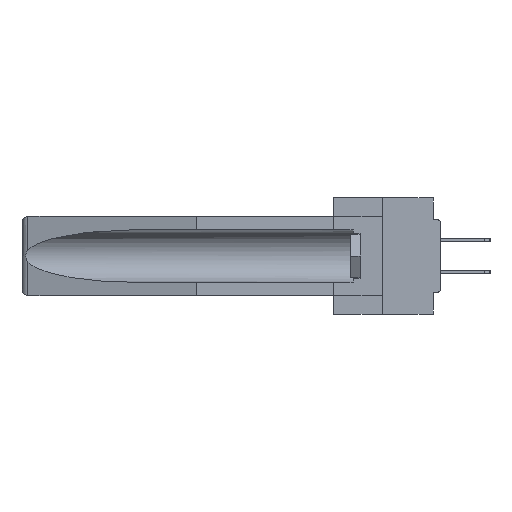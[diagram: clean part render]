
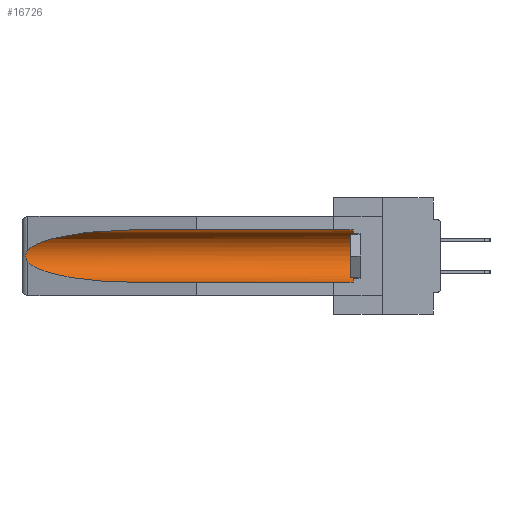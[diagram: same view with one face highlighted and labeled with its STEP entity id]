
A CAD part, left-side view. The second image highlights one B-rep face of the part: STEP entity #16726.
In plain terms, the highlighted cylindrical face has radius 2.857 mm (diameter 5.715 mm), a partial arc.
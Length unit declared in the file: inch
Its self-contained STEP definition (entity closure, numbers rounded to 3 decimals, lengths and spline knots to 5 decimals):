
#1860 = CARTESIAN_POINT ( 'NONE',  ( 0.2675, 1.53308, -0.16763 ) ) ;
#2304 = DIRECTION ( 'NONE',  ( 0., 1., 0. ) ) ;
#3188 = CARTESIAN_POINT ( 'NONE',  ( 0.25451, 1.48313, -0.09465 ) ) ;
#3666 = CARTESIAN_POINT ( 'NONE',  ( 0.155, 1.07973, -0.059 ) ) ;
#4475 = CARTESIAN_POINT ( 'NONE',  ( 0.26537, 1.52718, -0.19328 ) ) ;
#4611 = CARTESIAN_POINT ( 'NONE',  ( 0.26537, 1.52718, -0.14972 ) ) ;
#4769 = VERTEX_POINT ( 'NONE', #35009 ) ;
#4998 = AXIS2_PLACEMENT_3D ( 'NONE', #13197, #9573, #36963 ) ;
#6229 =( BOUNDED_CURVE ( )  B_SPLINE_CURVE ( 3, ( #36138, #35714, #3188, #15961 ),
 .UNSPECIFIED., .F., .F. ) 
 B_SPLINE_CURVE_WITH_KNOTS ( ( 4, 4 ),
 ( 4.71239, 6.08839 ),
 .UNSPECIFIED. ) 
 CURVE ( )  GEOMETRIC_REPRESENTATION_ITEM ( )  RATIONAL_B_SPLINE_CURVE ( ( 1., 0.848, 0.848, 1. ) ) 
 REPRESENTATION_ITEM ( '' )  );
#6712 = DIRECTION ( 'NONE',  ( 0., -1., 0. ) ) ;
#7484 = LINE ( 'NONE', #21594, #15284 ) ;
#8739 = VERTEX_POINT ( 'NONE', #35648 ) ;
#9002 = CARTESIAN_POINT ( 'NONE',  ( 0.21114, 1.30732, -0.284 ) ) ;
#9573 = DIRECTION ( 'NONE',  ( 0., 1., 0. ) ) ;
#9753 = ORIENTED_EDGE ( 'NONE', *, *, #20040, .T. ) ;
#10214 =( BOUNDED_CURVE ( )  B_SPLINE_CURVE ( 3, ( #25278, #19764, #9002, #38895 ),
 .UNSPECIFIED., .F., .F. ) 
 B_SPLINE_CURVE_WITH_KNOTS ( ( 4, 4 ),
 ( 0.1948, 1.5708 ),
 .UNSPECIFIED. ) 
 CURVE ( )  GEOMETRIC_REPRESENTATION_ITEM ( )  RATIONAL_B_SPLINE_CURVE ( ( 1., 0.848, 0.848, 1. ) ) 
 REPRESENTATION_ITEM ( '' )  );
#11291 = CARTESIAN_POINT ( 'NONE',  ( 0.2675, 1.53308, -0.17534 ) ) ;
#13197 = CARTESIAN_POINT ( 'NONE',  ( 0.155, -0.30754, -0.1715 ) ) ;
#14502 = ORIENTED_EDGE ( 'NONE', *, *, #35498, .T. ) ;
#15072 = CARTESIAN_POINT ( 'NONE',  ( 0.155, -0.30754, -0.059 ) ) ;
#15284 = VECTOR ( 'NONE', #37813, 39.37008 ) ;
#15778 = EDGE_LOOP ( 'NONE', ( #18957, #9753, #29349, #20083, #36887, #14502 ) ) ;
#15961 = CARTESIAN_POINT ( 'NONE',  ( 0.26537, 1.52718, -0.14972 ) ) ;
#16284 = EDGE_CURVE ( 'NONE', #30520, #24343, #24476, .T. ) ;
#16726 = ADVANCED_FACE ( 'NONE', ( #35346 ), #37397, .F. ) ;
#18957 = ORIENTED_EDGE ( 'NONE', *, *, #32190, .T. ) ;
#18969 = CARTESIAN_POINT ( 'NONE',  ( 0.155, 0.126, -0.284 ) ) ;
#19764 = CARTESIAN_POINT ( 'NONE',  ( 0.25451, 1.48313, -0.24835 ) ) ;
#20040 = EDGE_CURVE ( 'NONE', #4769, #8739, #41049, .T. ) ;
#20083 = ORIENTED_EDGE ( 'NONE', *, *, #35715, .F. ) ;
#21594 = CARTESIAN_POINT ( 'NONE',  ( 0.155, -0.30754, -0.284 ) ) ;
#24343 = VERTEX_POINT ( 'NONE', #40068 ) ;
#24476 = CIRCLE ( 'NONE', #41705, 0.1125 ) ;
#24818 = CARTESIAN_POINT ( 'NONE',  ( 0.26597, 1.5296, -0.19026 ) ) ;
#25278 = CARTESIAN_POINT ( 'NONE',  ( 0.26537, 1.52718, -0.19328 ) ) ;
#26588 = CARTESIAN_POINT ( 'NONE',  ( 0.155, 0.126, -0.1715 ) ) ;
#29349 = ORIENTED_EDGE ( 'NONE', *, *, #31550, .T. ) ;
#29413 = VERTEX_POINT ( 'NONE', #42694 ) ;
#29922 = DIRECTION ( 'NONE',  ( 0., 0., 1. ) ) ;
#30520 = VERTEX_POINT ( 'NONE', #18969 ) ;
#31341 = CARTESIAN_POINT ( 'NONE',  ( 0.2673, 1.53269, -0.17917 ) ) ;
#31491 = CARTESIAN_POINT ( 'NONE',  ( 0.26654, 1.53092, -0.15636 ) ) ;
#31550 = EDGE_CURVE ( 'NONE', #8739, #29413, #10214, .T. ) ;
#32190 = EDGE_CURVE ( 'NONE', #40282, #4769, #6229, .T. ) ;
#32474 = LINE ( 'NONE', #15072, #40699 ) ;
#34662 = CARTESIAN_POINT ( 'NONE',  ( 0.26655, 1.53094, -0.18657 ) ) ;
#35009 = CARTESIAN_POINT ( 'NONE',  ( 0.26537, 1.52718, -0.14972 ) ) ;
#35346 = FACE_OUTER_BOUND ( 'NONE', #15778, .T. ) ;
#35498 = EDGE_CURVE ( 'NONE', #24343, #40282, #32474, .T. ) ;
#35648 = CARTESIAN_POINT ( 'NONE',  ( 0.26537, 1.52718, -0.19328 ) ) ;
#35714 = CARTESIAN_POINT ( 'NONE',  ( 0.21114, 1.30732, -0.059 ) ) ;
#35715 = EDGE_CURVE ( 'NONE', #30520, #29413, #7484, .T. ) ;
#36138 = CARTESIAN_POINT ( 'NONE',  ( 0.155, 1.07973, -0.059 ) ) ;
#36887 = ORIENTED_EDGE ( 'NONE', *, *, #16284, .T. ) ;
#36963 = DIRECTION ( 'NONE',  ( 0., 0., 1. ) ) ;
#37397 = CYLINDRICAL_SURFACE ( 'NONE', #4998, 0.1125 ) ;
#37813 = DIRECTION ( 'NONE',  ( 0., 1., 0. ) ) ;
#37838 = CARTESIAN_POINT ( 'NONE',  ( 0.26597, 1.52961, -0.15275 ) ) ;
#38895 = CARTESIAN_POINT ( 'NONE',  ( 0.155, 1.07973, -0.284 ) ) ;
#40068 = CARTESIAN_POINT ( 'NONE',  ( 0.155, 0.126, -0.059 ) ) ;
#40282 = VERTEX_POINT ( 'NONE', #3666 ) ;
#40699 = VECTOR ( 'NONE', #2304, 39.37008 ) ;
#41045 = CARTESIAN_POINT ( 'NONE',  ( 0.2673, 1.5327, -0.16383 ) ) ;
#41049 = B_SPLINE_CURVE_WITH_KNOTS ( 'NONE', 3,
 ( #4611, #37838, #31491, #41045, #1860, #11291, #31341, #34662, #24818, #4475 ),
 .UNSPECIFIED., .F., .F.,
 ( 4, 2, 2, 2, 4 ),
 ( 0., 0.00029, 0.00058, 0.00087, 0.00117 ),
 .UNSPECIFIED. ) ;
#41705 = AXIS2_PLACEMENT_3D ( 'NONE', #26588, #6712, #29922 ) ;
#42694 = CARTESIAN_POINT ( 'NONE',  ( 0.155, 1.07973, -0.284 ) ) ;
